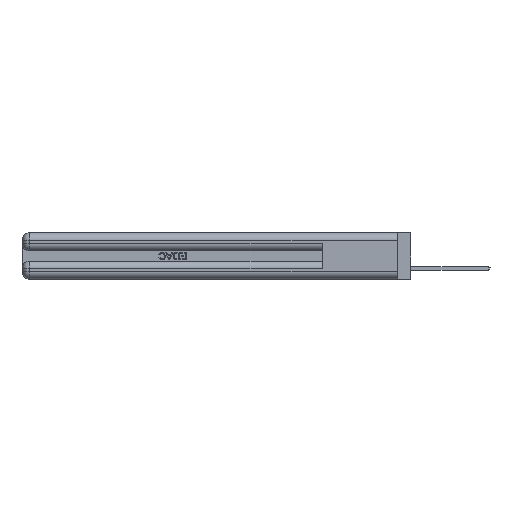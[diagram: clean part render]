
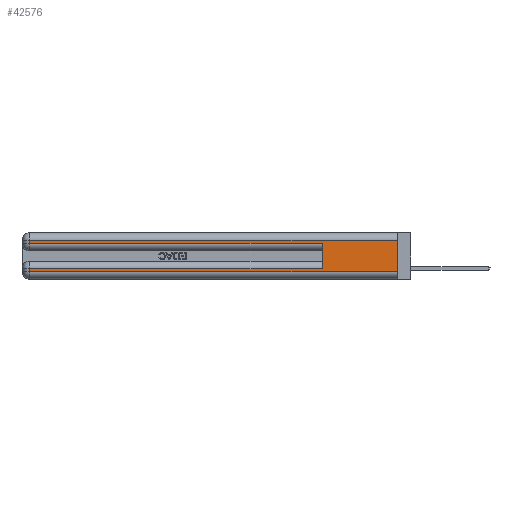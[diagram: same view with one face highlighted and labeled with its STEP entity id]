
A CAD part, left-side view. The second image highlights one B-rep face of the part: STEP entity #42576.
In plain terms, the highlighted planar face has unit normal (-1, 0, 0).
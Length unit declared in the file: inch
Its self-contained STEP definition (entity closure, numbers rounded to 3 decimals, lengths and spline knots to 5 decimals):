
#137 = CARTESIAN_POINT ( 'NONE',  ( 0., 0., 0.37 ) ) ;
#1811 = LINE ( 'NONE', #26155, #21586 ) ;
#2595 = LINE ( 'NONE', #39389, #34737 ) ;
#2723 = CARTESIAN_POINT ( 'NONE',  ( 0., 2.94, 0.06 ) ) ;
#3002 = DIRECTION ( 'NONE',  ( 0., 0., -1. ) ) ;
#5051 = LINE ( 'NONE', #137, #12817 ) ;
#5736 = FACE_OUTER_BOUND ( 'NONE', #19448, .T. ) ;
#5776 = ORIENTED_EDGE ( 'NONE', *, *, #6051, .T. ) ;
#6051 = EDGE_CURVE ( 'NONE', #32818, #29877, #46800, .T. ) ;
#6296 = CARTESIAN_POINT ( 'NONE',  ( 0., 2.94, 0.285 ) ) ;
#8379 = VECTOR ( 'NONE', #15984, 39.37008 ) ;
#8710 = CARTESIAN_POINT ( 'NONE',  ( 0., 0.6, 0.145 ) ) ;
#8957 = DIRECTION ( 'NONE',  ( 1., 0., 0. ) ) ;
#9533 = CARTESIAN_POINT ( 'NONE',  ( 0., 2.94, 0.085 ) ) ;
#10443 = DIRECTION ( 'NONE',  ( 0., -1., 0. ) ) ;
#10508 = EDGE_CURVE ( 'NONE', #12530, #32818, #1811, .T. ) ;
#11195 = CARTESIAN_POINT ( 'NONE',  ( 0., 0., 0.06 ) ) ;
#12530 = VERTEX_POINT ( 'NONE', #9533 ) ;
#12817 = VECTOR ( 'NONE', #26751, 39.37008 ) ;
#14229 = CARTESIAN_POINT ( 'NONE',  ( 0., 0., 0.31 ) ) ;
#14549 = VECTOR ( 'NONE', #35363, 39.37008 ) ;
#14581 = CARTESIAN_POINT ( 'NONE',  ( 0., 2.94, 0.31 ) ) ;
#15950 = ORIENTED_EDGE ( 'NONE', *, *, #16782, .T. ) ;
#15984 = DIRECTION ( 'NONE',  ( 0., 0., -1. ) ) ;
#16426 = VECTOR ( 'NONE', #18680, 39.37008 ) ;
#16782 = EDGE_CURVE ( 'NONE', #24574, #17636, #19370, .T. ) ;
#16794 = LINE ( 'NONE', #24007, #8379 ) ;
#17636 = VERTEX_POINT ( 'NONE', #44820 ) ;
#18175 = LINE ( 'NONE', #45558, #34799 ) ;
#18680 = DIRECTION ( 'NONE',  ( 0., -1., 0. ) ) ;
#19370 = LINE ( 'NONE', #37420, #40837 ) ;
#19448 = EDGE_LOOP ( 'NONE', ( #23274, #40951, #31070, #15950, #41548, #26558, #31405, #5776 ) ) ;
#21586 = VECTOR ( 'NONE', #3002, 39.37008 ) ;
#22800 = DIRECTION ( 'NONE',  ( 0., 1., 0. ) ) ;
#23274 = ORIENTED_EDGE ( 'NONE', *, *, #43129, .F. ) ;
#24007 = CARTESIAN_POINT ( 'NONE',  ( 0., 2.94, 0.37 ) ) ;
#24574 = VERTEX_POINT ( 'NONE', #6296 ) ;
#24803 = DIRECTION ( 'NONE',  ( 0., 0., -1. ) ) ;
#26155 = CARTESIAN_POINT ( 'NONE',  ( 0., 2.94, 0.37 ) ) ;
#26558 = ORIENTED_EDGE ( 'NONE', *, *, #38406, .T. ) ;
#26751 = DIRECTION ( 'NONE',  ( 0., 0., -1. ) ) ;
#28268 = PLANE ( 'NONE',  #30683 ) ;
#29877 = VERTEX_POINT ( 'NONE', #43296 ) ;
#30683 = AXIS2_PLACEMENT_3D ( 'NONE', #35955, #8957, #24803 ) ;
#30894 = VERTEX_POINT ( 'NONE', #14581 ) ;
#31070 = ORIENTED_EDGE ( 'NONE', *, *, #39422, .T. ) ;
#31335 = VERTEX_POINT ( 'NONE', #14229 ) ;
#31405 = ORIENTED_EDGE ( 'NONE', *, *, #10508, .T. ) ;
#32818 = VERTEX_POINT ( 'NONE', #2723 ) ;
#33603 = LINE ( 'NONE', #8710, #14549 ) ;
#34737 = VECTOR ( 'NONE', #44258, 39.37008 ) ;
#34799 = VECTOR ( 'NONE', #22800, 39.37008 ) ;
#35363 = DIRECTION ( 'NONE',  ( 0., 0., 1. ) ) ;
#35955 = CARTESIAN_POINT ( 'NONE',  ( 0., 0., 0.37 ) ) ;
#37404 = CARTESIAN_POINT ( 'NONE',  ( 0., 0.6, 0.085 ) ) ;
#37420 = CARTESIAN_POINT ( 'NONE',  ( 0., 0., 0.285 ) ) ;
#38036 = VERTEX_POINT ( 'NONE', #37404 ) ;
#38406 = EDGE_CURVE ( 'NONE', #38036, #12530, #2595, .T. ) ;
#39389 = CARTESIAN_POINT ( 'NONE',  ( 0., 0., 0.085 ) ) ;
#39422 = EDGE_CURVE ( 'NONE', #30894, #24574, #16794, .T. ) ;
#40837 = VECTOR ( 'NONE', #10443, 39.37008 ) ;
#40951 = ORIENTED_EDGE ( 'NONE', *, *, #45829, .T. ) ;
#41548 = ORIENTED_EDGE ( 'NONE', *, *, #45983, .F. ) ;
#42576 = ADVANCED_FACE ( 'NONE', ( #5736 ), #28268, .F. ) ;
#43129 = EDGE_CURVE ( 'NONE', #31335, #29877, #5051, .T. ) ;
#43296 = CARTESIAN_POINT ( 'NONE',  ( 0., 0., 0.06 ) ) ;
#44258 = DIRECTION ( 'NONE',  ( 0., 1., 0. ) ) ;
#44820 = CARTESIAN_POINT ( 'NONE',  ( 0., 0.6, 0.285 ) ) ;
#45558 = CARTESIAN_POINT ( 'NONE',  ( 0., 0., 0.31 ) ) ;
#45829 = EDGE_CURVE ( 'NONE', #31335, #30894, #18175, .T. ) ;
#45983 = EDGE_CURVE ( 'NONE', #38036, #17636, #33603, .T. ) ;
#46800 = LINE ( 'NONE', #11195, #16426 ) ;
